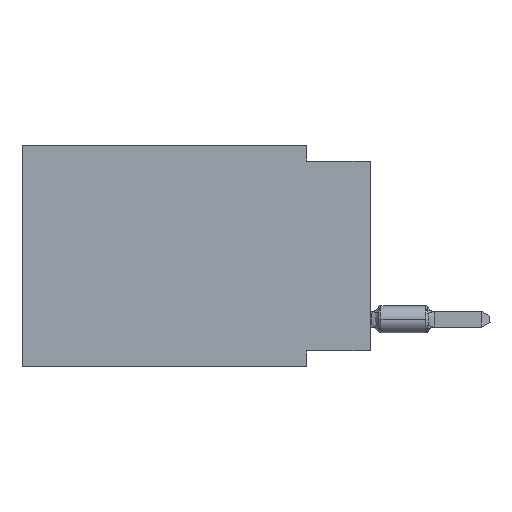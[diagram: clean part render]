
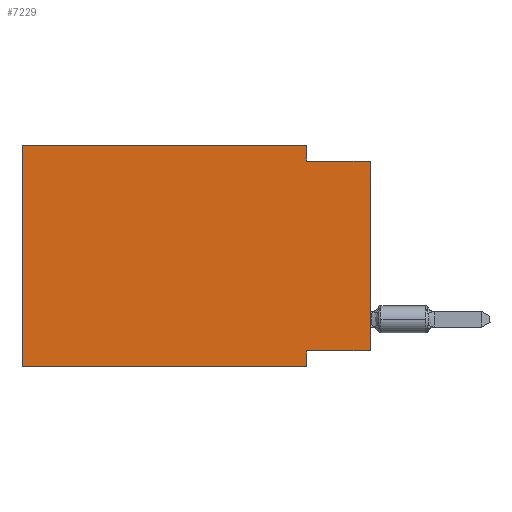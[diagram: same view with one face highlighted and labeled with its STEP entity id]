
A CAD part, left-side view. The second image highlights one B-rep face of the part: STEP entity #7229.
In plain terms, the highlighted planar face has unit normal (-1, 0, 0).
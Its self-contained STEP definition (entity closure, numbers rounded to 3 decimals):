
#10 = VECTOR ( 'NONE', #8186, 1000. ) ;
#27 = VECTOR ( 'NONE', #11929, 1000. ) ;
#368 = LINE ( 'NONE', #12716, #4218 ) ;
#909 = EDGE_CURVE ( 'NONE', #4263, #5576, #12776, .T. ) ;
#1023 = LINE ( 'NONE', #5148, #10138 ) ;
#1078 = VECTOR ( 'NONE', #12844, 1000. ) ;
#1448 = PLANE ( 'NONE',  #13123 ) ;
#1503 = CARTESIAN_POINT ( 'NONE',  ( 0., 0., 0. ) ) ;
#1796 = CARTESIAN_POINT ( 'NONE',  ( 0., 13.97, -8.89 ) ) ;
#1934 = EDGE_CURVE ( 'NONE', #12206, #12540, #4703, .T. ) ;
#2282 = ORIENTED_EDGE ( 'NONE', *, *, #6569, .T. ) ;
#2479 = EDGE_CURVE ( 'NONE', #4263, #12520, #1023, .T. ) ;
#2555 = DIRECTION ( 'NONE',  ( 0., 0., -1. ) ) ;
#2576 = CARTESIAN_POINT ( 'NONE',  ( 0., 2.54, -0.635 ) ) ;
#2992 = VERTEX_POINT ( 'NONE', #3431 ) ;
#3170 = VECTOR ( 'NONE', #8030, 1000. ) ;
#3431 = CARTESIAN_POINT ( 'NONE',  ( 0., 2.54, 0. ) ) ;
#4218 = VECTOR ( 'NONE', #4368, 1000. ) ;
#4263 = VERTEX_POINT ( 'NONE', #6102 ) ;
#4320 = VECTOR ( 'NONE', #12045, 1000. ) ;
#4368 = DIRECTION ( 'NONE',  ( 0., -1., 0. ) ) ;
#4564 = CARTESIAN_POINT ( 'NONE',  ( 0., 13.97, 0. ) ) ;
#4623 = CARTESIAN_POINT ( 'NONE',  ( 0., 13.97, 0. ) ) ;
#4703 = LINE ( 'NONE', #11057, #27 ) ;
#4708 = VERTEX_POINT ( 'NONE', #2576 ) ;
#4863 = CARTESIAN_POINT ( 'NONE',  ( 0., 2.54, -8.255 ) ) ;
#5117 = CARTESIAN_POINT ( 'NONE',  ( 0., 2.54, -8.89 ) ) ;
#5148 = CARTESIAN_POINT ( 'NONE',  ( 0., 0., -8.255 ) ) ;
#5576 = VERTEX_POINT ( 'NONE', #10122 ) ;
#5652 = DIRECTION ( 'NONE',  ( 1., 0., 0. ) ) ;
#6089 = CARTESIAN_POINT ( 'NONE',  ( 0., 13.97, -8.89 ) ) ;
#6102 = CARTESIAN_POINT ( 'NONE',  ( 0., 0., -8.255 ) ) ;
#6333 = ORIENTED_EDGE ( 'NONE', *, *, #12637, .F. ) ;
#6569 = EDGE_CURVE ( 'NONE', #12206, #7892, #7824, .T. ) ;
#6691 = ORIENTED_EDGE ( 'NONE', *, *, #2479, .F. ) ;
#6753 = ORIENTED_EDGE ( 'NONE', *, *, #9756, .F. ) ;
#7111 = LINE ( 'NONE', #5117, #10 ) ;
#7229 = ADVANCED_FACE ( 'NONE', ( #9526 ), #1448, .F. ) ;
#7248 = EDGE_CURVE ( 'NONE', #4708, #5576, #368, .T. ) ;
#7824 = LINE ( 'NONE', #1796, #3170 ) ;
#7892 = VERTEX_POINT ( 'NONE', #12141 ) ;
#8030 = DIRECTION ( 'NONE',  ( 0., -1., 0. ) ) ;
#8186 = DIRECTION ( 'NONE',  ( 0., 0., -1. ) ) ;
#8250 = ORIENTED_EDGE ( 'NONE', *, *, #909, .T. ) ;
#9279 = ORIENTED_EDGE ( 'NONE', *, *, #1934, .F. ) ;
#9526 = FACE_OUTER_BOUND ( 'NONE', #9638, .T. ) ;
#9638 = EDGE_LOOP ( 'NONE', ( #8250, #9695, #6753, #10397, #9279, #2282, #6333, #6691 ) ) ;
#9695 = ORIENTED_EDGE ( 'NONE', *, *, #7248, .F. ) ;
#9756 = EDGE_CURVE ( 'NONE', #2992, #4708, #13033, .T. ) ;
#9836 = CARTESIAN_POINT ( 'NONE',  ( 0., 2.54, 0. ) ) ;
#10044 = DIRECTION ( 'NONE',  ( 0., 0., -1. ) ) ;
#10122 = CARTESIAN_POINT ( 'NONE',  ( 0., 0., -0.635 ) ) ;
#10138 = VECTOR ( 'NONE', #10262, 1000. ) ;
#10262 = DIRECTION ( 'NONE',  ( 0., 1., 0. ) ) ;
#10397 = ORIENTED_EDGE ( 'NONE', *, *, #13249, .F. ) ;
#11057 = CARTESIAN_POINT ( 'NONE',  ( 0., 13.97, 0. ) ) ;
#11463 = VECTOR ( 'NONE', #10044, 1000. ) ;
#11929 = DIRECTION ( 'NONE',  ( 0., 0., 1. ) ) ;
#12045 = DIRECTION ( 'NONE',  ( 0., -1., 0. ) ) ;
#12141 = CARTESIAN_POINT ( 'NONE',  ( 0., 2.54, -8.89 ) ) ;
#12206 = VERTEX_POINT ( 'NONE', #6089 ) ;
#12520 = VERTEX_POINT ( 'NONE', #4863 ) ;
#12540 = VERTEX_POINT ( 'NONE', #12944 ) ;
#12637 = EDGE_CURVE ( 'NONE', #12520, #7892, #7111, .T. ) ;
#12716 = CARTESIAN_POINT ( 'NONE',  ( 0., 0., -0.635 ) ) ;
#12776 = LINE ( 'NONE', #1503, #1078 ) ;
#12844 = DIRECTION ( 'NONE',  ( 0., 0., 1. ) ) ;
#12944 = CARTESIAN_POINT ( 'NONE',  ( 0., 13.97, 0. ) ) ;
#13033 = LINE ( 'NONE', #9836, #11463 ) ;
#13055 = LINE ( 'NONE', #4564, #4320 ) ;
#13123 = AXIS2_PLACEMENT_3D ( 'NONE', #4623, #5652, #2555 ) ;
#13249 = EDGE_CURVE ( 'NONE', #12540, #2992, #13055, .T. ) ;
